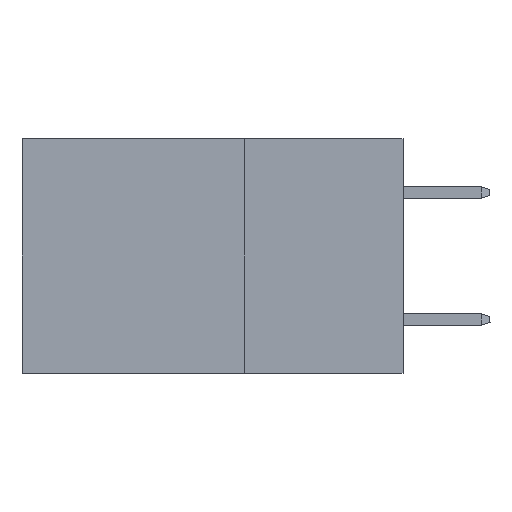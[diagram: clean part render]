
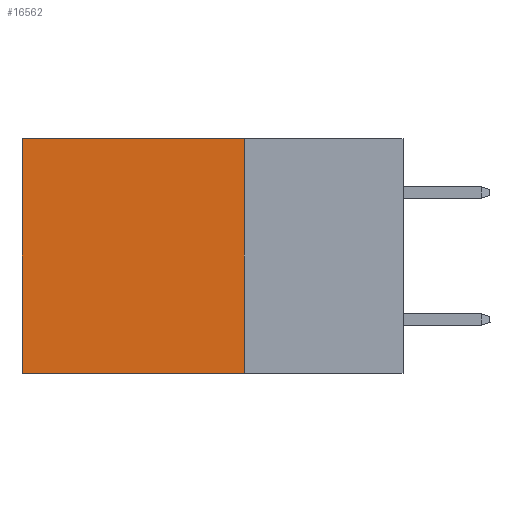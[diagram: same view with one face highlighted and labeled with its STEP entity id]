
A CAD part, left-side view. The second image highlights one B-rep face of the part: STEP entity #16562.
In plain terms, the highlighted planar face has unit normal (-1, 0, 0).
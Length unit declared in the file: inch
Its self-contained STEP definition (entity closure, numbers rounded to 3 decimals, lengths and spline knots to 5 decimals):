
#1309 = VERTEX_POINT ( 'NONE', #27621 ) ;
#1765 = VERTEX_POINT ( 'NONE', #16797 ) ;
#1838 = ORIENTED_EDGE ( 'NONE', *, *, #25745, .F. ) ;
#1981 = ORIENTED_EDGE ( 'NONE', *, *, #22499, .T. ) ;
#2224 = LINE ( 'NONE', #23378, #6376 ) ;
#2481 = LINE ( 'NONE', #23312, #3145 ) ;
#2736 = VECTOR ( 'NONE', #4899, 39.37008 ) ;
#3145 = VECTOR ( 'NONE', #21039, 39.37008 ) ;
#3932 = DIRECTION ( 'NONE',  ( 0., 1., 0. ) ) ;
#4899 = DIRECTION ( 'NONE',  ( 0., 1., 0. ) ) ;
#6376 = VECTOR ( 'NONE', #31094, 39.37008 ) ;
#6830 = LINE ( 'NONE', #14514, #24288 ) ;
#6841 = DIRECTION ( 'NONE',  ( 0., 0., -1. ) ) ;
#9577 = FACE_OUTER_BOUND ( 'NONE', #27319, .T. ) ;
#12059 = LINE ( 'NONE', #19904, #2736 ) ;
#13177 = ORIENTED_EDGE ( 'NONE', *, *, #20934, .T. ) ;
#14514 = CARTESIAN_POINT ( 'NONE',  ( 0.2875, 0.25, -0.37 ) ) ;
#16562 = ADVANCED_FACE ( 'NONE', ( #9577 ), #22005, .F. ) ;
#16565 = CARTESIAN_POINT ( 'NONE',  ( 0.2875, 0.25, 0. ) ) ;
#16797 = CARTESIAN_POINT ( 'NONE',  ( 0.2875, 0.6, 0. ) ) ;
#17062 = DIRECTION ( 'NONE',  ( 1., 0., 0. ) ) ;
#18098 = EDGE_CURVE ( 'NONE', #22846, #1309, #2224, .T. ) ;
#19904 = CARTESIAN_POINT ( 'NONE',  ( 0.2875, 0.25, 0. ) ) ;
#20049 = CARTESIAN_POINT ( 'NONE',  ( 0.2875, 0.25, 0. ) ) ;
#20934 = EDGE_CURVE ( 'NONE', #22846, #1765, #12059, .T. ) ;
#21039 = DIRECTION ( 'NONE',  ( 0., 0., -1. ) ) ;
#22005 = PLANE ( 'NONE',  #31038 ) ;
#22499 = EDGE_CURVE ( 'NONE', #1765, #30560, #2481, .T. ) ;
#22846 = VERTEX_POINT ( 'NONE', #20049 ) ;
#23312 = CARTESIAN_POINT ( 'NONE',  ( 0.2875, 0.6, 0. ) ) ;
#23378 = CARTESIAN_POINT ( 'NONE',  ( 0.2875, 0.25, 0. ) ) ;
#24288 = VECTOR ( 'NONE', #3932, 39.37008 ) ;
#25745 = EDGE_CURVE ( 'NONE', #1309, #30560, #6830, .T. ) ;
#27319 = EDGE_LOOP ( 'NONE', ( #1981, #1838, #31676, #13177 ) ) ;
#27621 = CARTESIAN_POINT ( 'NONE',  ( 0.2875, 0.25, -0.37 ) ) ;
#30560 = VERTEX_POINT ( 'NONE', #32525 ) ;
#31038 = AXIS2_PLACEMENT_3D ( 'NONE', #16565, #17062, #6841 ) ;
#31094 = DIRECTION ( 'NONE',  ( 0., 0., -1. ) ) ;
#31676 = ORIENTED_EDGE ( 'NONE', *, *, #18098, .F. ) ;
#32525 = CARTESIAN_POINT ( 'NONE',  ( 0.2875, 0.6, -0.37 ) ) ;
